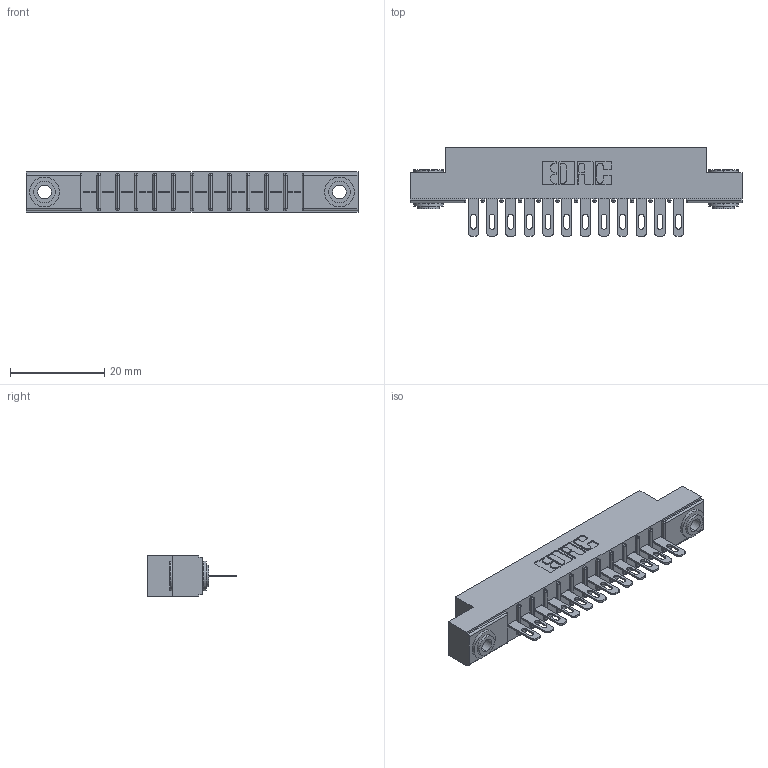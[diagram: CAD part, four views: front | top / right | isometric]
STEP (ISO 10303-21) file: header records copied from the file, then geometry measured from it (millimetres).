
FILE_DESCRIPTION (( 'STEP AP203' ), '1' );
FILE_NAME ('306-012-500-103.STEP', '2019-09-11T19:30:07', ( '' ), ( '' ), 'SwSTEP 2.0', 'SolidWorks 2016', '' );
FILE_SCHEMA (( 'CONFIG_CONTROL_DESIGN' ));
Length unit declared in the file: inch
Products named in the file (4): 306-012-500-103; 306-290-001_100; 306 Part_.156 Dia; 345-250-002_345-250-002-102
Assembly tree (15 placements, depth 2):
  306-012-500-103
    306 Part_.156 Dia
    306-290-001_100  x12
    345-250-002_345-250-002-102  x2
Bounding box: 70.56 x 18.87 x 8.71 mm (x, y, z)
Volume: 4817.6 mm3; surface area: 7260.7 mm2
Topology: 15 solids, 15 shells, 1080 faces, 3008 edges, 1936 vertices
Faces by surface type: plane 692, cylinder 332, sphere 48, cone 8
Entity records: 16306 total; most frequent: CARTESIAN_POINT 2712, DIRECTION 2692, ORIENTED_EDGE 2676, EDGE_CURVE 1338, VECTOR 1020, LINE 1020, VERTEX_POINT 856, AXIS2_PLACEMENT_3D 836
